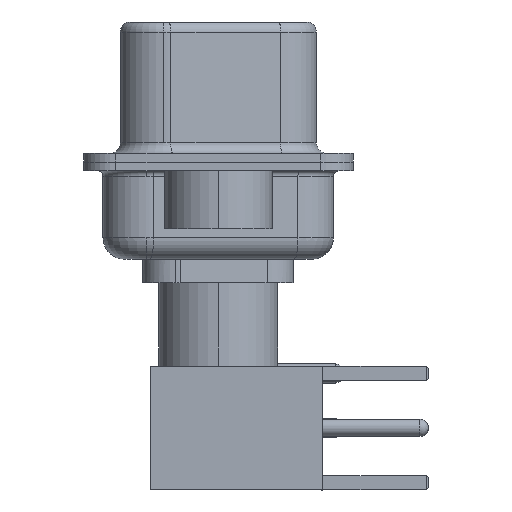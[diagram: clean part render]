
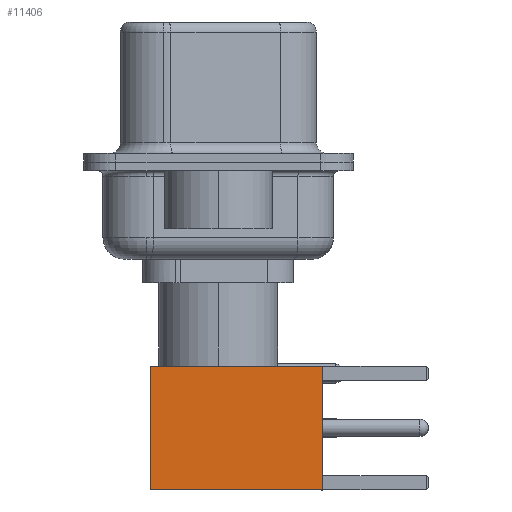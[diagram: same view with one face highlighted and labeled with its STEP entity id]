
A CAD part, left-side view. The second image highlights one B-rep face of the part: STEP entity #11406.
In plain terms, the highlighted face is planar.
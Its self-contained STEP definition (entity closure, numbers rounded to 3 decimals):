
#863 = CARTESIAN_POINT ( 'NONE',  ( 2.875, 2.875, 0. ) ) ;
#1136 = VERTEX_POINT ( 'NONE', #12178 ) ;
#2035 = VECTOR ( 'NONE', #18611, 1000. ) ;
#2676 = DIRECTION ( 'NONE',  ( 0., 0., -1. ) ) ;
#6384 = EDGE_CURVE ( 'NONE', #17213, #7700, #30040, .T. ) ;
#6446 = CARTESIAN_POINT ( 'NONE',  ( 0., 2.875, 0. ) ) ;
#6459 = EDGE_CURVE ( 'NONE', #1136, #7700, #13918, .T. ) ;
#7285 = VECTOR ( 'NONE', #18017, 1000. ) ;
#7700 = VERTEX_POINT ( 'NONE', #25119 ) ;
#9585 = ORIENTED_EDGE ( 'NONE', *, *, #6459, .F. ) ;
#10103 = LINE ( 'NONE', #863, #10252 ) ;
#10252 = VECTOR ( 'NONE', #26982, 1000. ) ;
#11406 = ADVANCED_FACE ( 'NONE', ( #27941 ), #20906, .T. ) ;
#12017 = ORIENTED_EDGE ( 'NONE', *, *, #30519, .F. ) ;
#12178 = CARTESIAN_POINT ( 'NONE',  ( -2.875, 2.875, 8. ) ) ;
#13399 = CARTESIAN_POINT ( 'NONE',  ( 2.875, 2.875, 0. ) ) ;
#13918 = LINE ( 'NONE', #26427, #30001 ) ;
#15396 = ORIENTED_EDGE ( 'NONE', *, *, #28458, .T. ) ;
#15522 = LINE ( 'NONE', #26954, #7285 ) ;
#17213 = VERTEX_POINT ( 'NONE', #21322 ) ;
#17734 = VERTEX_POINT ( 'NONE', #30861 ) ;
#18017 = DIRECTION ( 'NONE',  ( -1., 0., 0. ) ) ;
#18611 = DIRECTION ( 'NONE',  ( -1., 0., 0. ) ) ;
#20906 = PLANE ( 'NONE',  #27420 ) ;
#21322 = CARTESIAN_POINT ( 'NONE',  ( 2.875, 2.875, 0. ) ) ;
#21834 = EDGE_LOOP ( 'NONE', ( #15396, #22172, #9585, #12017 ) ) ;
#22172 = ORIENTED_EDGE ( 'NONE', *, *, #6384, .T. ) ;
#22952 = DIRECTION ( 'NONE',  ( 0., 0., 1. ) ) ;
#25119 = CARTESIAN_POINT ( 'NONE',  ( -2.875, 2.875, 0. ) ) ;
#26427 = CARTESIAN_POINT ( 'NONE',  ( -2.875, 2.875, 0. ) ) ;
#26954 = CARTESIAN_POINT ( 'NONE',  ( 0., 2.875, 8. ) ) ;
#26982 = DIRECTION ( 'NONE',  ( 0., 0., -1. ) ) ;
#27420 = AXIS2_PLACEMENT_3D ( 'NONE', #13399, #28102, #22952 ) ;
#27941 = FACE_OUTER_BOUND ( 'NONE', #21834, .T. ) ;
#28102 = DIRECTION ( 'NONE',  ( 0., 1., 0. ) ) ;
#28458 = EDGE_CURVE ( 'NONE', #17734, #17213, #10103, .T. ) ;
#30001 = VECTOR ( 'NONE', #2676, 1000. ) ;
#30040 = LINE ( 'NONE', #6446, #2035 ) ;
#30519 = EDGE_CURVE ( 'NONE', #17734, #1136, #15522, .T. ) ;
#30861 = CARTESIAN_POINT ( 'NONE',  ( 2.875, 2.875, 8. ) ) ;
